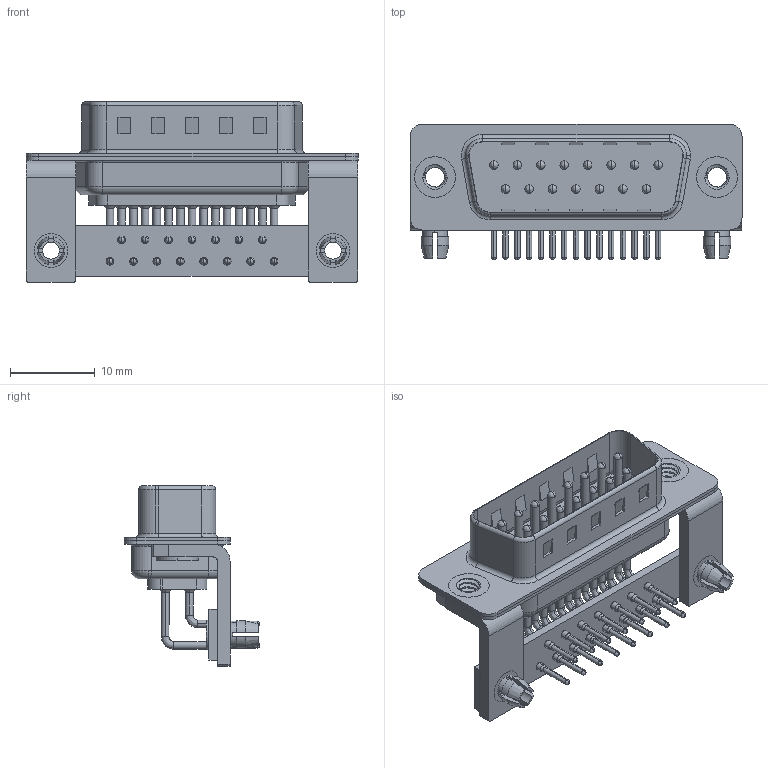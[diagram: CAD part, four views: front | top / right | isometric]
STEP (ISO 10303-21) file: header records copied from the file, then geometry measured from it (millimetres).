
FILE_DESCRIPTION (( 'STEP AP203' ), '1' );
FILE_NAME ('629-M15-240-LN3.STEP', '2018-09-25T17:11:09', ( '' ), ( '' ), 'SwSTEP 2.0', 'SolidWorks 2016', '' );
FILE_SCHEMA (( 'CONFIG_CONTROL_DESIGN' ));
Length unit declared in the file: millimetre
Products named in the file (10): 629M Board Lock; 629M Housing_15 Contacts; 629-M15-240-LN3; 629M Shell Front_15 Contacts; 629M Shell Rear_15 Contacts; 629M Contact Row 1; 629M Contact Row 2; 629M 4-40 Threaded Rivet_Stabilizer; 629M Stabilizer Bracket; 629M Stabilizer Board_15 Contacts
Assembly tree (25 placements, depth 2):
  629-M15-240-LN3
    629M Housing_15 Contacts
    629M Shell Front_15 Contacts
    629M Shell Rear_15 Contacts
    629M Contact Row 1  x8
    629M Contact Row 2  x7
    629M 4-40 Threaded Rivet_Stabilizer  x2
    629M Stabilizer Bracket  x2
    629M Stabilizer Board_15 Contacts
    629M Board Lock  x2
Bounding box: 39.2 x 16 x 21.3 mm (x, y, z)
Volume: 2481 mm3; surface area: 6762.4 mm2
Topology: 25 solids, 25 shells, 2162 faces, 5989 edges, 3892 vertices
Faces by surface type: plane 1173, cylinder 757, bspline 96, cone 80, torus 56
Entity records: 25996 total; most frequent: CARTESIAN_POINT 5643, DIRECTION 4121, ORIENTED_EDGE 3828, EDGE_CURVE 1914, AXIS2_PLACEMENT_3D 1508, VERTEX_POINT 1240, LINE 1105, VECTOR 1105
